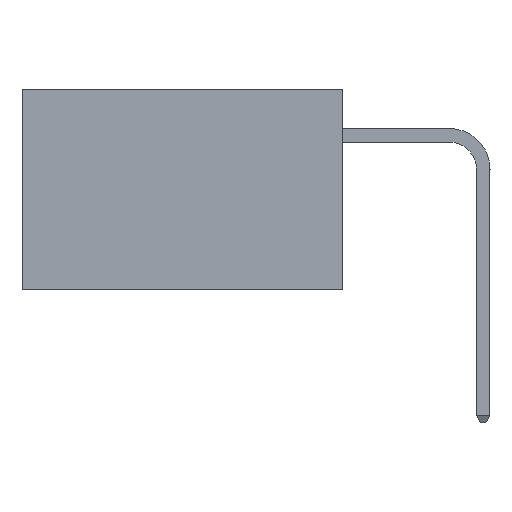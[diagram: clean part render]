
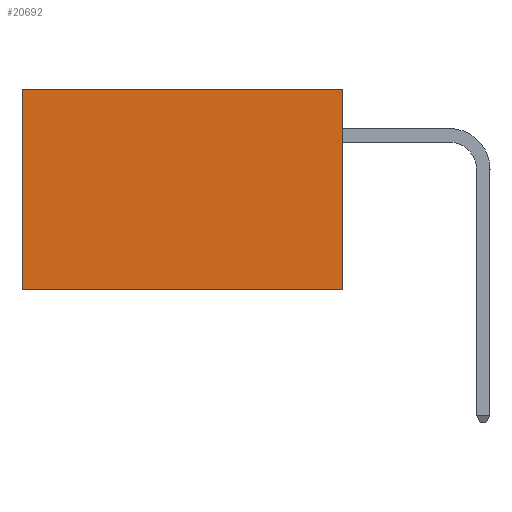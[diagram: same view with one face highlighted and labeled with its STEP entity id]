
A CAD part, left-side view. The second image highlights one B-rep face of the part: STEP entity #20692.
In plain terms, the highlighted planar face has unit normal (-1, 0, 0).
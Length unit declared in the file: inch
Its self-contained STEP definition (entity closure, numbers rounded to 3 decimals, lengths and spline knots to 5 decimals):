
#143 = ORIENTED_EDGE ( 'NONE', *, *, #6799, .F. ) ;
#1150 = AXIS2_PLACEMENT_3D ( 'NONE', #21740, #8004, #21814 ) ;
#1208 = VERTEX_POINT ( 'NONE', #22286 ) ;
#1815 = VERTEX_POINT ( 'NONE', #17908 ) ;
#2184 = LINE ( 'NONE', #21473, #8072 ) ;
#3781 = CARTESIAN_POINT ( 'NONE',  ( 0.277, 0., -0.37 ) ) ;
#3858 = EDGE_LOOP ( 'NONE', ( #3873, #19098, #143, #11593 ) ) ;
#3873 = ORIENTED_EDGE ( 'NONE', *, *, #22316, .T. ) ;
#4215 = DIRECTION ( 'NONE',  ( 0., 0., -1. ) ) ;
#4270 = CARTESIAN_POINT ( 'NONE',  ( 0.277, 0., -0.37 ) ) ;
#5232 = LINE ( 'NONE', #11824, #15827 ) ;
#6038 = PLANE ( 'NONE',  #1150 ) ;
#6317 = VECTOR ( 'NONE', #4215, 39.37008 ) ;
#6799 = EDGE_CURVE ( 'NONE', #1208, #12519, #16887, .T. ) ;
#7643 = DIRECTION ( 'NONE',  ( 0., 1., 0. ) ) ;
#8004 = DIRECTION ( 'NONE',  ( 1., 0., 0. ) ) ;
#8072 = VECTOR ( 'NONE', #7643, 39.37008 ) ;
#8808 = EDGE_CURVE ( 'NONE', #1208, #1815, #14607, .T. ) ;
#9880 = DIRECTION ( 'NONE',  ( 0., 1., 0. ) ) ;
#10028 = CARTESIAN_POINT ( 'NONE',  ( 0.277, 0., 0. ) ) ;
#10347 = VERTEX_POINT ( 'NONE', #11471 ) ;
#11471 = CARTESIAN_POINT ( 'NONE',  ( 0.277, 0.59, -0.37 ) ) ;
#11593 = ORIENTED_EDGE ( 'NONE', *, *, #8808, .T. ) ;
#11824 = CARTESIAN_POINT ( 'NONE',  ( 0.277, 0.59, -0.37 ) ) ;
#12519 = VERTEX_POINT ( 'NONE', #3781 ) ;
#14607 = LINE ( 'NONE', #10028, #24278 ) ;
#15827 = VECTOR ( 'NONE', #25340, 39.37008 ) ;
#16887 = LINE ( 'NONE', #4270, #6317 ) ;
#17908 = CARTESIAN_POINT ( 'NONE',  ( 0.277, 0.59, 0. ) ) ;
#19098 = ORIENTED_EDGE ( 'NONE', *, *, #19277, .F. ) ;
#19277 = EDGE_CURVE ( 'NONE', #12519, #10347, #2184, .T. ) ;
#20692 = ADVANCED_FACE ( 'NONE', ( #23361 ), #6038, .F. ) ;
#21473 = CARTESIAN_POINT ( 'NONE',  ( 0.277, 0., -0.37 ) ) ;
#21740 = CARTESIAN_POINT ( 'NONE',  ( 0.277, 0., -0.37 ) ) ;
#21814 = DIRECTION ( 'NONE',  ( 0., 0., -1. ) ) ;
#22286 = CARTESIAN_POINT ( 'NONE',  ( 0.277, 0., 0. ) ) ;
#22316 = EDGE_CURVE ( 'NONE', #1815, #10347, #5232, .T. ) ;
#23361 = FACE_OUTER_BOUND ( 'NONE', #3858, .T. ) ;
#24278 = VECTOR ( 'NONE', #9880, 39.37008 ) ;
#25340 = DIRECTION ( 'NONE',  ( 0., 0., -1. ) ) ;
